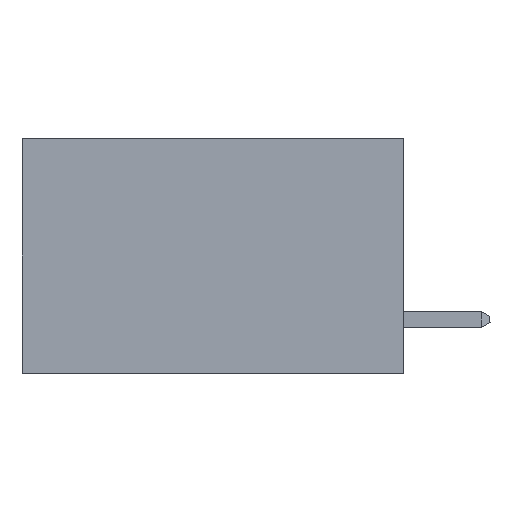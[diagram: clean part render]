
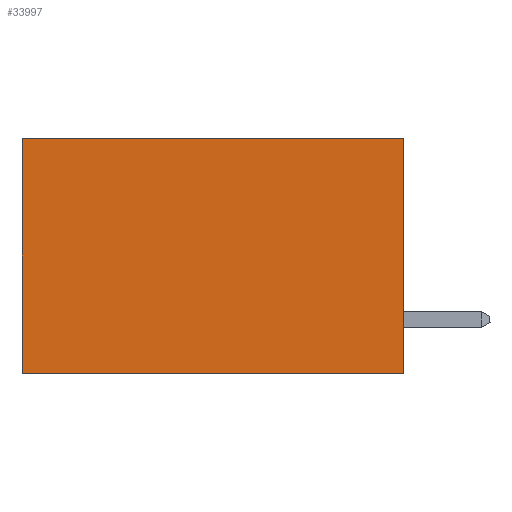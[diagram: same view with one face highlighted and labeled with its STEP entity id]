
A CAD part, left-side view. The second image highlights one B-rep face of the part: STEP entity #33997.
In plain terms, the highlighted planar face has unit normal (-1, 0, 0).
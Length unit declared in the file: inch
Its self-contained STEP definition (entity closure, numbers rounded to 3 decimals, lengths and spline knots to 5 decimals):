
#3926 = EDGE_CURVE ( 'NONE', #36797, #16673, #43921, .T. ) ;
#4364 = AXIS2_PLACEMENT_3D ( 'NONE', #21071, #36531, #36869 ) ;
#8078 = VECTOR ( 'NONE', #21203, 39.37008 ) ;
#8837 = EDGE_CURVE ( 'NONE', #10181, #9530, #19954, .T. ) ;
#9530 = VERTEX_POINT ( 'NONE', #41531 ) ;
#10033 = VECTOR ( 'NONE', #22377, 39.37008 ) ;
#10181 = VERTEX_POINT ( 'NONE', #33731 ) ;
#10414 = CARTESIAN_POINT ( 'NONE',  ( 0.2875, 0., -0.37 ) ) ;
#11477 = ORIENTED_EDGE ( 'NONE', *, *, #8837, .F. ) ;
#14330 = PLANE ( 'NONE',  #4364 ) ;
#15138 = EDGE_CURVE ( 'NONE', #36797, #10181, #17045, .T. ) ;
#16673 = VERTEX_POINT ( 'NONE', #36715 ) ;
#17045 = LINE ( 'NONE', #35603, #8078 ) ;
#17196 = EDGE_CURVE ( 'NONE', #16673, #9530, #22511, .T. ) ;
#18892 = CARTESIAN_POINT ( 'NONE',  ( 0.2875, 0., 0. ) ) ;
#19954 = LINE ( 'NONE', #10414, #27651 ) ;
#20504 = CARTESIAN_POINT ( 'NONE',  ( 0.2875, 0.6, 0. ) ) ;
#21071 = CARTESIAN_POINT ( 'NONE',  ( 0.2875, 0., 0. ) ) ;
#21203 = DIRECTION ( 'NONE',  ( 0., 0., -1. ) ) ;
#22377 = DIRECTION ( 'NONE',  ( 0., 1., 0. ) ) ;
#22511 = LINE ( 'NONE', #20504, #41564 ) ;
#27651 = VECTOR ( 'NONE', #43250, 39.37008 ) ;
#27825 = FACE_OUTER_BOUND ( 'NONE', #31674, .T. ) ;
#28383 = CARTESIAN_POINT ( 'NONE',  ( 0.2875, 0., 0. ) ) ;
#29563 = ORIENTED_EDGE ( 'NONE', *, *, #15138, .F. ) ;
#31674 = EDGE_LOOP ( 'NONE', ( #38733, #11477, #29563, #45630 ) ) ;
#33731 = CARTESIAN_POINT ( 'NONE',  ( 0.2875, 0., -0.37 ) ) ;
#33997 = ADVANCED_FACE ( 'NONE', ( #27825 ), #14330, .F. ) ;
#35603 = CARTESIAN_POINT ( 'NONE',  ( 0.2875, 0., 0. ) ) ;
#36531 = DIRECTION ( 'NONE',  ( 1., 0., 0. ) ) ;
#36715 = CARTESIAN_POINT ( 'NONE',  ( 0.2875, 0.6, 0. ) ) ;
#36797 = VERTEX_POINT ( 'NONE', #28383 ) ;
#36869 = DIRECTION ( 'NONE',  ( 0., 0., -1. ) ) ;
#38733 = ORIENTED_EDGE ( 'NONE', *, *, #17196, .T. ) ;
#39529 = DIRECTION ( 'NONE',  ( 0., 0., -1. ) ) ;
#41531 = CARTESIAN_POINT ( 'NONE',  ( 0.2875, 0.6, -0.37 ) ) ;
#41564 = VECTOR ( 'NONE', #39529, 39.37008 ) ;
#43250 = DIRECTION ( 'NONE',  ( 0., 1., 0. ) ) ;
#43921 = LINE ( 'NONE', #18892, #10033 ) ;
#45630 = ORIENTED_EDGE ( 'NONE', *, *, #3926, .T. ) ;
